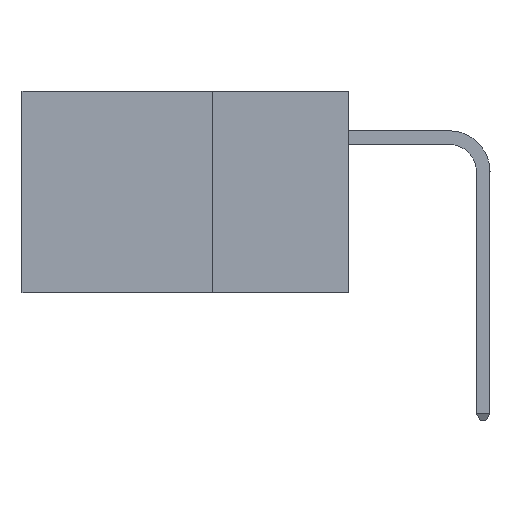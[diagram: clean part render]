
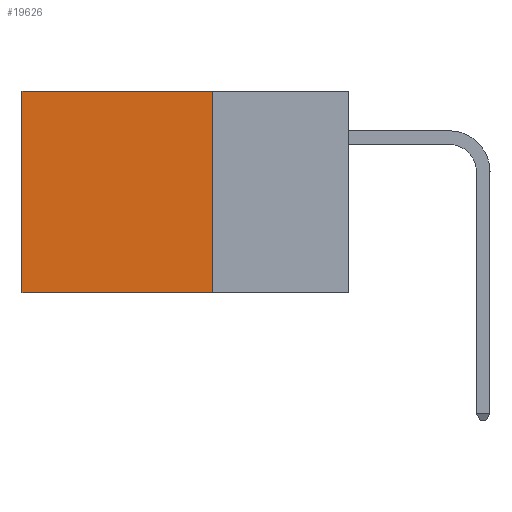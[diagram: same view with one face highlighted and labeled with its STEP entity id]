
A CAD part, left-side view. The second image highlights one B-rep face of the part: STEP entity #19626.
In plain terms, the highlighted planar face has unit normal (-1, 0, 0).
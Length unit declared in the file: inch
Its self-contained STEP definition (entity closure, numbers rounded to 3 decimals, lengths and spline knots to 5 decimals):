
#549 = DIRECTION ( 'NONE',  ( 0., 0., -1. ) ) ;
#2133 = CARTESIAN_POINT ( 'NONE',  ( 0.2875, 0.25, 0. ) ) ;
#2866 = EDGE_CURVE ( 'NONE', #18104, #31154, #27064, .T. ) ;
#5584 = EDGE_LOOP ( 'NONE', ( #26455, #6980, #10382, #15643 ) ) ;
#6980 = ORIENTED_EDGE ( 'NONE', *, *, #20759, .F. ) ;
#7039 = CARTESIAN_POINT ( 'NONE',  ( 0.2875, 0.25, -0.37 ) ) ;
#8969 = CARTESIAN_POINT ( 'NONE',  ( 0.2875, 0.25, 0. ) ) ;
#9219 = CARTESIAN_POINT ( 'NONE',  ( 0.2875, 0.25, 0. ) ) ;
#10382 = ORIENTED_EDGE ( 'NONE', *, *, #2866, .F. ) ;
#11055 = CARTESIAN_POINT ( 'NONE',  ( 0.2875, 0.6, 0. ) ) ;
#11079 = VECTOR ( 'NONE', #17769, 39.37008 ) ;
#12170 = VERTEX_POINT ( 'NONE', #11055 ) ;
#12225 = VERTEX_POINT ( 'NONE', #18450 ) ;
#12713 = PLANE ( 'NONE',  #13360 ) ;
#13066 = FACE_OUTER_BOUND ( 'NONE', #5584, .T. ) ;
#13360 = AXIS2_PLACEMENT_3D ( 'NONE', #29844, #15162, #549 ) ;
#14042 = VECTOR ( 'NONE', #26351, 39.37008 ) ;
#15162 = DIRECTION ( 'NONE',  ( 1., 0., 0. ) ) ;
#15289 = CARTESIAN_POINT ( 'NONE',  ( 0.2875, 0.25, -0.37 ) ) ;
#15643 = ORIENTED_EDGE ( 'NONE', *, *, #17452, .T. ) ;
#16953 = VECTOR ( 'NONE', #25241, 39.37008 ) ;
#17452 = EDGE_CURVE ( 'NONE', #18104, #12170, #27323, .T. ) ;
#17753 = LINE ( 'NONE', #25140, #16953 ) ;
#17769 = DIRECTION ( 'NONE',  ( 0., 1., 0. ) ) ;
#18104 = VERTEX_POINT ( 'NONE', #2133 ) ;
#18450 = CARTESIAN_POINT ( 'NONE',  ( 0.2875, 0.6, -0.37 ) ) ;
#19626 = ADVANCED_FACE ( 'NONE', ( #13066 ), #12713, .F. ) ;
#20085 = VECTOR ( 'NONE', #21304, 39.37008 ) ;
#20759 = EDGE_CURVE ( 'NONE', #31154, #12225, #30641, .T. ) ;
#21304 = DIRECTION ( 'NONE',  ( 0., 1., 0. ) ) ;
#25140 = CARTESIAN_POINT ( 'NONE',  ( 0.2875, 0.6, 0. ) ) ;
#25241 = DIRECTION ( 'NONE',  ( 0., 0., -1. ) ) ;
#26226 = EDGE_CURVE ( 'NONE', #12170, #12225, #17753, .T. ) ;
#26351 = DIRECTION ( 'NONE',  ( 0., 0., -1. ) ) ;
#26455 = ORIENTED_EDGE ( 'NONE', *, *, #26226, .T. ) ;
#27064 = LINE ( 'NONE', #9219, #14042 ) ;
#27323 = LINE ( 'NONE', #8969, #20085 ) ;
#29844 = CARTESIAN_POINT ( 'NONE',  ( 0.2875, 0.25, 0. ) ) ;
#30641 = LINE ( 'NONE', #15289, #11079 ) ;
#31154 = VERTEX_POINT ( 'NONE', #7039 ) ;
